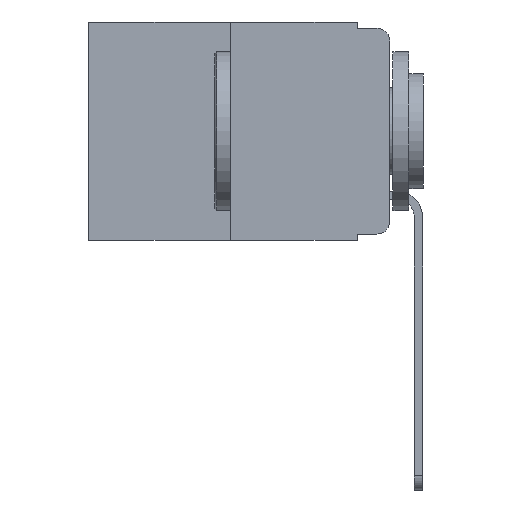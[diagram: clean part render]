
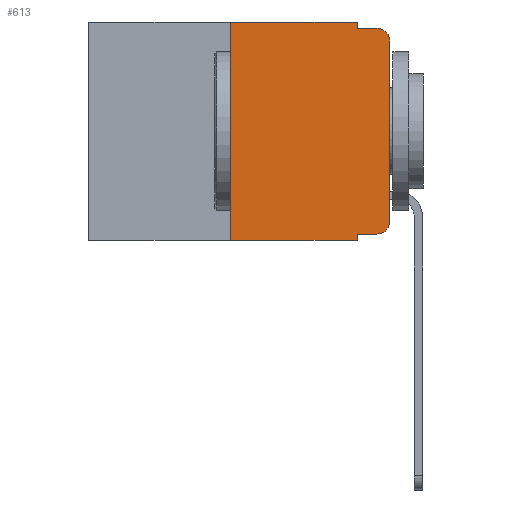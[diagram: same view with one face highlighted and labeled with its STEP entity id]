
A CAD part, left-side view. The second image highlights one B-rep face of the part: STEP entity #613.
In plain terms, the highlighted planar face has unit normal (-1, 0, 0).
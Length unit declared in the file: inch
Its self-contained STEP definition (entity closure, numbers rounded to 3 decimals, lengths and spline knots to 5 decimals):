
#8 = ORIENTED_EDGE ( 'NONE', *, *, #16926, .F. ) ;
#268 = ORIENTED_EDGE ( 'NONE', *, *, #14168, .T. ) ;
#477 = ORIENTED_EDGE ( 'NONE', *, *, #6937, .T. ) ;
#524 = ORIENTED_EDGE ( 'NONE', *, *, #13253, .T. ) ;
#547 = CARTESIAN_POINT ( 'NONE',  ( 0., 0.25, 0. ) ) ;
#613 = ADVANCED_FACE ( 'NONE', ( #16208 ), #8457, .F. ) ;
#628 = ORIENTED_EDGE ( 'NONE', *, *, #17797, .F. ) ;
#644 = ORIENTED_EDGE ( 'NONE', *, *, #15564, .F. ) ;
#815 = EDGE_CURVE ( 'NONE', #17876, #16684, #14932, .T. ) ;
#823 = VERTEX_POINT ( 'NONE', #5867 ) ;
#884 = LINE ( 'NONE', #15736, #1384 ) ;
#968 = ORIENTED_EDGE ( 'NONE', *, *, #16026, .F. ) ;
#1252 = LINE ( 'NONE', #16396, #6103 ) ;
#1286 = VERTEX_POINT ( 'NONE', #4139 ) ;
#1384 = VECTOR ( 'NONE', #3500, 39.37008 ) ;
#1461 = LINE ( 'NONE', #15221, #12928 ) ;
#1844 = CIRCLE ( 'NONE', #7551, 0.02 ) ;
#1996 = LINE ( 'NONE', #13039, #9720 ) ;
#2698 = DIRECTION ( 'NONE',  ( 0., -1., 0. ) ) ;
#2829 = LINE ( 'NONE', #18535, #17714 ) ;
#2958 = EDGE_CURVE ( 'NONE', #10795, #17876, #884, .T. ) ;
#3500 = DIRECTION ( 'NONE',  ( 0., 0., 1. ) ) ;
#3590 = DIRECTION ( 'NONE',  ( 0., -1., 0. ) ) ;
#3884 = CARTESIAN_POINT ( 'NONE',  ( 0., 0.02, -0.313 ) ) ;
#4139 = CARTESIAN_POINT ( 'NONE',  ( 0., 0.051, -0.333 ) ) ;
#4811 = VERTEX_POINT ( 'NONE', #547 ) ;
#4936 = DIRECTION ( 'NONE',  ( 0., 0., -1. ) ) ;
#5444 = CARTESIAN_POINT ( 'NONE',  ( 0., 0.02, -0.333 ) ) ;
#5542 = DIRECTION ( 'NONE',  ( 0., 0., -1. ) ) ;
#5867 = CARTESIAN_POINT ( 'NONE',  ( 0., 0.051, -0.01 ) ) ;
#6103 = VECTOR ( 'NONE', #6667, 39.37008 ) ;
#6204 = ORIENTED_EDGE ( 'NONE', *, *, #2958, .T. ) ;
#6229 = ORIENTED_EDGE ( 'NONE', *, *, #815, .T. ) ;
#6667 = DIRECTION ( 'NONE',  ( 0., 0., -1. ) ) ;
#6742 = DIRECTION ( 'NONE',  ( 0., 0., 1. ) ) ;
#6937 = EDGE_CURVE ( 'NONE', #9384, #18301, #13445, .T. ) ;
#7551 = AXIS2_PLACEMENT_3D ( 'NONE', #3884, #14066, #5542 ) ;
#8179 = CARTESIAN_POINT ( 'NONE',  ( 0., 0.25, 0. ) ) ;
#8253 = EDGE_LOOP ( 'NONE', ( #6204, #6229, #14277, #628, #644, #8, #477, #968, #268, #524 ) ) ;
#8409 = DIRECTION ( 'NONE',  ( 0., 0., -1. ) ) ;
#8457 = PLANE ( 'NONE',  #15386 ) ;
#8503 = CARTESIAN_POINT ( 'NONE',  ( 0., 0., -0.313 ) ) ;
#8630 = LINE ( 'NONE', #17942, #12730 ) ;
#9384 = VERTEX_POINT ( 'NONE', #13420 ) ;
#9467 = AXIS2_PLACEMENT_3D ( 'NONE', #17158, #18166, #15492 ) ;
#9720 = VECTOR ( 'NONE', #11620, 39.37008 ) ;
#10352 = LINE ( 'NONE', #8179, #17253 ) ;
#10795 = VERTEX_POINT ( 'NONE', #8503 ) ;
#11620 = DIRECTION ( 'NONE',  ( 0., -1., 0. ) ) ;
#12291 = DIRECTION ( 'NONE',  ( 1., 0., 0. ) ) ;
#12571 = DIRECTION ( 'NONE',  ( 0., -1., 0. ) ) ;
#12634 = CARTESIAN_POINT ( 'NONE',  ( 0., 0.473, -0.343 ) ) ;
#12730 = VECTOR ( 'NONE', #8409, 39.37008 ) ;
#12928 = VECTOR ( 'NONE', #3590, 39.37008 ) ;
#13005 = VECTOR ( 'NONE', #12571, 39.37008 ) ;
#13039 = CARTESIAN_POINT ( 'NONE',  ( 0., 0.473, 0. ) ) ;
#13253 = EDGE_CURVE ( 'NONE', #16286, #10795, #1844, .T. ) ;
#13420 = CARTESIAN_POINT ( 'NONE',  ( 0., 0.25, -0.343 ) ) ;
#13445 = LINE ( 'NONE', #12634, #13005 ) ;
#14027 = CARTESIAN_POINT ( 'NONE',  ( 0., 0., -0.03 ) ) ;
#14066 = DIRECTION ( 'NONE',  ( -1., 0., 0. ) ) ;
#14168 = EDGE_CURVE ( 'NONE', #1286, #16286, #2829, .T. ) ;
#14277 = ORIENTED_EDGE ( 'NONE', *, *, #18674, .F. ) ;
#14727 = CARTESIAN_POINT ( 'NONE',  ( 0., 0.02, -0.01 ) ) ;
#14932 = CIRCLE ( 'NONE', #9467, 0.02 ) ;
#14988 = CARTESIAN_POINT ( 'NONE',  ( 0., 0.051, 0. ) ) ;
#15221 = CARTESIAN_POINT ( 'NONE',  ( 0., 0.051, -0.01 ) ) ;
#15386 = AXIS2_PLACEMENT_3D ( 'NONE', #17321, #12291, #4936 ) ;
#15492 = DIRECTION ( 'NONE',  ( 0., 0., -1. ) ) ;
#15564 = EDGE_CURVE ( 'NONE', #4811, #18508, #1996, .T. ) ;
#15736 = CARTESIAN_POINT ( 'NONE',  ( 0., 0., 0. ) ) ;
#16026 = EDGE_CURVE ( 'NONE', #1286, #18301, #1252, .T. ) ;
#16208 = FACE_OUTER_BOUND ( 'NONE', #8253, .T. ) ;
#16286 = VERTEX_POINT ( 'NONE', #5444 ) ;
#16396 = CARTESIAN_POINT ( 'NONE',  ( 0., 0.051, 0. ) ) ;
#16684 = VERTEX_POINT ( 'NONE', #14727 ) ;
#16926 = EDGE_CURVE ( 'NONE', #9384, #4811, #10352, .T. ) ;
#17158 = CARTESIAN_POINT ( 'NONE',  ( 0., 0.02, -0.03 ) ) ;
#17253 = VECTOR ( 'NONE', #6742, 39.37008 ) ;
#17321 = CARTESIAN_POINT ( 'NONE',  ( 0., 0.473, 0. ) ) ;
#17412 = CARTESIAN_POINT ( 'NONE',  ( 0., 0.051, -0.343 ) ) ;
#17714 = VECTOR ( 'NONE', #2698, 39.37008 ) ;
#17797 = EDGE_CURVE ( 'NONE', #18508, #823, #8630, .T. ) ;
#17876 = VERTEX_POINT ( 'NONE', #14027 ) ;
#17942 = CARTESIAN_POINT ( 'NONE',  ( 0., 0.051, 0. ) ) ;
#18166 = DIRECTION ( 'NONE',  ( -1., 0., 0. ) ) ;
#18301 = VERTEX_POINT ( 'NONE', #17412 ) ;
#18508 = VERTEX_POINT ( 'NONE', #14988 ) ;
#18535 = CARTESIAN_POINT ( 'NONE',  ( 0., 0.051, -0.333 ) ) ;
#18674 = EDGE_CURVE ( 'NONE', #823, #16684, #1461, .T. ) ;
